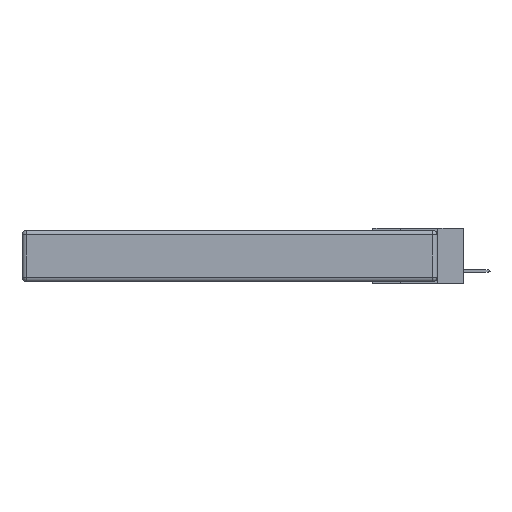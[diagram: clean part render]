
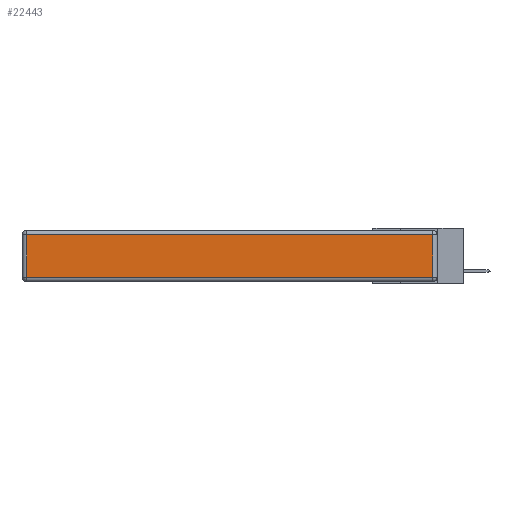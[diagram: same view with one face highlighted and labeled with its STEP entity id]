
A CAD part, left-side view. The second image highlights one B-rep face of the part: STEP entity #22443.
In plain terms, the highlighted planar face has unit normal (-1, 0, 0).
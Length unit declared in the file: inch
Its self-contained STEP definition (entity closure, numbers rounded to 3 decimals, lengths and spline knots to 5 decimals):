
#595 = EDGE_LOOP ( 'NONE', ( #11590, #21494, #4959, #778 ) ) ;
#778 = ORIENTED_EDGE ( 'NONE', *, *, #26513, .T. ) ;
#2052 = LINE ( 'NONE', #21493, #2835 ) ;
#2282 = PLANE ( 'NONE',  #30048 ) ;
#2835 = VECTOR ( 'NONE', #9122, 39.37008 ) ;
#3154 = LINE ( 'NONE', #19875, #18789 ) ;
#3189 = EDGE_CURVE ( 'NONE', #16179, #14258, #3154, .T. ) ;
#4959 = ORIENTED_EDGE ( 'NONE', *, *, #15000, .T. ) ;
#5042 = CARTESIAN_POINT ( 'NONE',  ( 0., 0., -0.343 ) ) ;
#5698 = LINE ( 'NONE', #20569, #18533 ) ;
#8368 = EDGE_CURVE ( 'NONE', #14258, #16912, #2052, .T. ) ;
#8486 = DIRECTION ( 'NONE',  ( 0., 0., -1. ) ) ;
#9066 = FACE_OUTER_BOUND ( 'NONE', #595, .T. ) ;
#9122 = DIRECTION ( 'NONE',  ( 0., 0., 1. ) ) ;
#9691 = DIRECTION ( 'NONE',  ( -1., 0., 0. ) ) ;
#10388 = VECTOR ( 'NONE', #8486, 39.37008 ) ;
#11590 = ORIENTED_EDGE ( 'NONE', *, *, #3189, .T. ) ;
#13144 = DIRECTION ( 'NONE',  ( 0., -1., 0. ) ) ;
#14258 = VERTEX_POINT ( 'NONE', #15653 ) ;
#14684 = CARTESIAN_POINT ( 'NONE',  ( 0., 2.72, -0.313 ) ) ;
#15000 = EDGE_CURVE ( 'NONE', #16912, #23951, #5698, .T. ) ;
#15653 = CARTESIAN_POINT ( 'NONE',  ( 0., 0.03, -0.313 ) ) ;
#16179 = VERTEX_POINT ( 'NONE', #14684 ) ;
#16912 = VERTEX_POINT ( 'NONE', #25297 ) ;
#18533 = VECTOR ( 'NONE', #23161, 39.37008 ) ;
#18789 = VECTOR ( 'NONE', #13144, 39.37008 ) ;
#19875 = CARTESIAN_POINT ( 'NONE',  ( 0., 0., -0.313 ) ) ;
#20569 = CARTESIAN_POINT ( 'NONE',  ( 0., 2.75, -0.03 ) ) ;
#21493 = CARTESIAN_POINT ( 'NONE',  ( 0., 0.03, -0.343 ) ) ;
#21494 = ORIENTED_EDGE ( 'NONE', *, *, #8368, .T. ) ;
#22443 = ADVANCED_FACE ( 'NONE', ( #9066 ), #2282, .T. ) ;
#23161 = DIRECTION ( 'NONE',  ( 0., 1., 0. ) ) ;
#23214 = CARTESIAN_POINT ( 'NONE',  ( 0., 2.72, -0.03 ) ) ;
#23668 = CARTESIAN_POINT ( 'NONE',  ( 0., 2.72, -0.343 ) ) ;
#23951 = VERTEX_POINT ( 'NONE', #23214 ) ;
#24502 = LINE ( 'NONE', #23668, #10388 ) ;
#25297 = CARTESIAN_POINT ( 'NONE',  ( 0., 0.03, -0.03 ) ) ;
#26513 = EDGE_CURVE ( 'NONE', #23951, #16179, #24502, .T. ) ;
#30048 = AXIS2_PLACEMENT_3D ( 'NONE', #5042, #9691, #32331 ) ;
#32331 = DIRECTION ( 'NONE',  ( 0., 0., 1. ) ) ;
